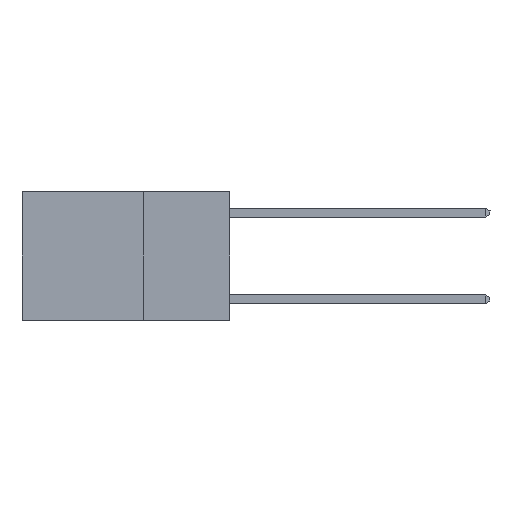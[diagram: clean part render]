
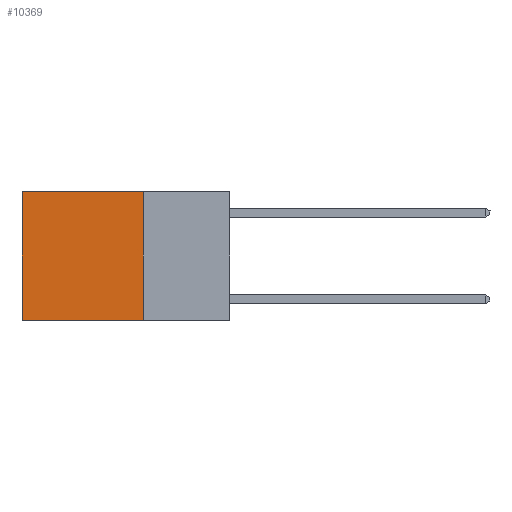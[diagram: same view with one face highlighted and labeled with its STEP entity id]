
A CAD part, left-side view. The second image highlights one B-rep face of the part: STEP entity #10369.
In plain terms, the highlighted planar face has unit normal (-1, 0, 0).
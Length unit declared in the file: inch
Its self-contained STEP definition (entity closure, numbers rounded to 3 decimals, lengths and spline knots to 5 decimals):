
#359 = VECTOR ( 'NONE', #15397, 39.37008 ) ;
#644 = VERTEX_POINT ( 'NONE', #24542 ) ;
#1361 = VECTOR ( 'NONE', #8223, 39.37008 ) ;
#1539 = CARTESIAN_POINT ( 'NONE',  ( 0.2625, 0.25, -0.37 ) ) ;
#2268 = CARTESIAN_POINT ( 'NONE',  ( 0.2625, 0.25, 0. ) ) ;
#2622 = VERTEX_POINT ( 'NONE', #15096 ) ;
#3062 = VERTEX_POINT ( 'NONE', #8653 ) ;
#3088 = DIRECTION ( 'NONE',  ( 0., 0., -1. ) ) ;
#3447 = ORIENTED_EDGE ( 'NONE', *, *, #22667, .T. ) ;
#4686 = FACE_OUTER_BOUND ( 'NONE', #24840, .T. ) ;
#5016 = CARTESIAN_POINT ( 'NONE',  ( 0.2625, 0.25, 0. ) ) ;
#6155 = CARTESIAN_POINT ( 'NONE',  ( 0.2625, 0.25, 0. ) ) ;
#6229 = CARTESIAN_POINT ( 'NONE',  ( 0.2625, 0.6, 0. ) ) ;
#7004 = VECTOR ( 'NONE', #12477, 39.37008 ) ;
#8223 = DIRECTION ( 'NONE',  ( 0., 0., -1. ) ) ;
#8653 = CARTESIAN_POINT ( 'NONE',  ( 0.2625, 0.6, 0. ) ) ;
#8940 = ORIENTED_EDGE ( 'NONE', *, *, #13234, .F. ) ;
#9013 = ORIENTED_EDGE ( 'NONE', *, *, #14377, .T. ) ;
#10369 = ADVANCED_FACE ( 'NONE', ( #4686 ), #22685, .F. ) ;
#10513 = CARTESIAN_POINT ( 'NONE',  ( 0.2625, 0.25, 0. ) ) ;
#11821 = VERTEX_POINT ( 'NONE', #2268 ) ;
#12477 = DIRECTION ( 'NONE',  ( 0., 0., -1. ) ) ;
#13158 = VECTOR ( 'NONE', #23825, 39.37008 ) ;
#13234 = EDGE_CURVE ( 'NONE', #11821, #2622, #22003, .T. ) ;
#14377 = EDGE_CURVE ( 'NONE', #3062, #644, #17071, .T. ) ;
#14905 = DIRECTION ( 'NONE',  ( 1., 0., 0. ) ) ;
#15096 = CARTESIAN_POINT ( 'NONE',  ( 0.2625, 0.25, -0.37 ) ) ;
#15099 = EDGE_CURVE ( 'NONE', #2622, #644, #21297, .T. ) ;
#15397 = DIRECTION ( 'NONE',  ( 0., 1., 0. ) ) ;
#15801 = AXIS2_PLACEMENT_3D ( 'NONE', #5016, #14905, #3088 ) ;
#17071 = LINE ( 'NONE', #6229, #1361 ) ;
#18711 = ORIENTED_EDGE ( 'NONE', *, *, #15099, .F. ) ;
#21297 = LINE ( 'NONE', #1539, #359 ) ;
#22003 = LINE ( 'NONE', #10513, #7004 ) ;
#22667 = EDGE_CURVE ( 'NONE', #11821, #3062, #25445, .T. ) ;
#22685 = PLANE ( 'NONE',  #15801 ) ;
#23825 = DIRECTION ( 'NONE',  ( 0., 1., 0. ) ) ;
#24542 = CARTESIAN_POINT ( 'NONE',  ( 0.2625, 0.6, -0.37 ) ) ;
#24840 = EDGE_LOOP ( 'NONE', ( #9013, #18711, #8940, #3447 ) ) ;
#25445 = LINE ( 'NONE', #6155, #13158 ) ;
